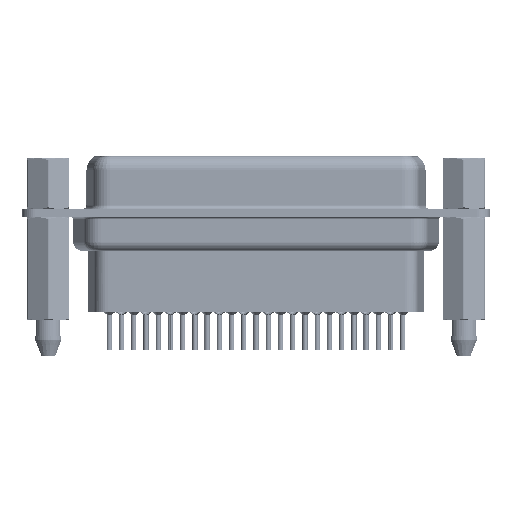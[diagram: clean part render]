
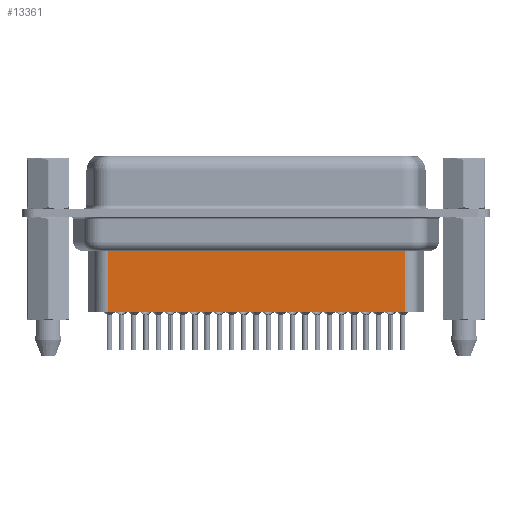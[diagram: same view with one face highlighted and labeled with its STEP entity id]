
A CAD part, front view. The second image highlights one B-rep face of the part: STEP entity #13361.
In plain terms, the highlighted planar face has unit normal (0, -1, 0).
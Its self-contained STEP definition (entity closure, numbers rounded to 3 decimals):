
#2510 = PLANE ( 'NONE',  #21997 ) ;
#5921 = VECTOR ( 'NONE', #28332, 1000. ) ;
#7181 = ORIENTED_EDGE ( 'NONE', *, *, #12879, .F. ) ;
#7207 = VERTEX_POINT ( 'NONE', #22642 ) ;
#7232 = CARTESIAN_POINT ( 'NONE',  ( 6.706, -3.5, -3.1 ) ) ;
#9356 = VECTOR ( 'NONE', #31076, 1000. ) ;
#9959 = EDGE_CURVE ( 'NONE', #25536, #27138, #30070, .T. ) ;
#10743 = CARTESIAN_POINT ( 'NONE',  ( 6.706, -3.5, -11.15 ) ) ;
#11980 = EDGE_LOOP ( 'NONE', ( #7181, #16816, #16324, #19227 ) ) ;
#12879 = EDGE_CURVE ( 'NONE', #7207, #27855, #28852, .T. ) ;
#13179 = FACE_OUTER_BOUND ( 'NONE', #11980, .T. ) ;
#13359 = LINE ( 'NONE', #10743, #15187 ) ;
#13361 = ADVANCED_FACE ( 'NONE', ( #13179 ), #2510, .T. ) ;
#13521 = DIRECTION ( 'NONE',  ( -1., 0., 0. ) ) ;
#14219 = VECTOR ( 'NONE', #19907, 1000. ) ;
#15187 = VECTOR ( 'NONE', #13521, 1000. ) ;
#16324 = ORIENTED_EDGE ( 'NONE', *, *, #9959, .T. ) ;
#16816 = ORIENTED_EDGE ( 'NONE', *, *, #21737, .T. ) ;
#17844 = LINE ( 'NONE', #31553, #5921 ) ;
#18136 = CARTESIAN_POINT ( 'NONE',  ( 6.706, -3.5, -4.097 ) ) ;
#18238 = CARTESIAN_POINT ( 'NONE',  ( 40.344, -3.5, -11.15 ) ) ;
#18314 = DIRECTION ( 'NONE',  ( 0., -1., 0. ) ) ;
#19227 = ORIENTED_EDGE ( 'NONE', *, *, #32825, .F. ) ;
#19907 = DIRECTION ( 'NONE',  ( 0., 0., -1. ) ) ;
#20543 = CARTESIAN_POINT ( 'NONE',  ( 6.706, -3.5, -11.15 ) ) ;
#21737 = EDGE_CURVE ( 'NONE', #7207, #25536, #17844, .T. ) ;
#21997 = AXIS2_PLACEMENT_3D ( 'NONE', #25723, #18314, #28815 ) ;
#22642 = CARTESIAN_POINT ( 'NONE',  ( 40.344, -3.5, -4.097 ) ) ;
#25536 = VERTEX_POINT ( 'NONE', #18136 ) ;
#25723 = CARTESIAN_POINT ( 'NONE',  ( 6.706, -3.5, -3.1 ) ) ;
#27138 = VERTEX_POINT ( 'NONE', #20543 ) ;
#27855 = VERTEX_POINT ( 'NONE', #18238 ) ;
#28332 = DIRECTION ( 'NONE',  ( -1., 0., 0. ) ) ;
#28815 = DIRECTION ( 'NONE',  ( 1., 0., 0. ) ) ;
#28852 = LINE ( 'NONE', #33654, #9356 ) ;
#30070 = LINE ( 'NONE', #7232, #14219 ) ;
#31076 = DIRECTION ( 'NONE',  ( 0., 0., -1. ) ) ;
#31553 = CARTESIAN_POINT ( 'NONE',  ( 6.459, -3.5, -4.097 ) ) ;
#32825 = EDGE_CURVE ( 'NONE', #27855, #27138, #13359, .T. ) ;
#33654 = CARTESIAN_POINT ( 'NONE',  ( 40.344, -3.5, -3.1 ) ) ;
